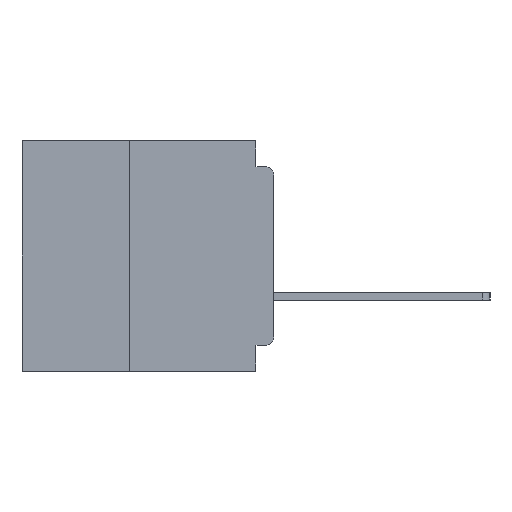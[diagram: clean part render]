
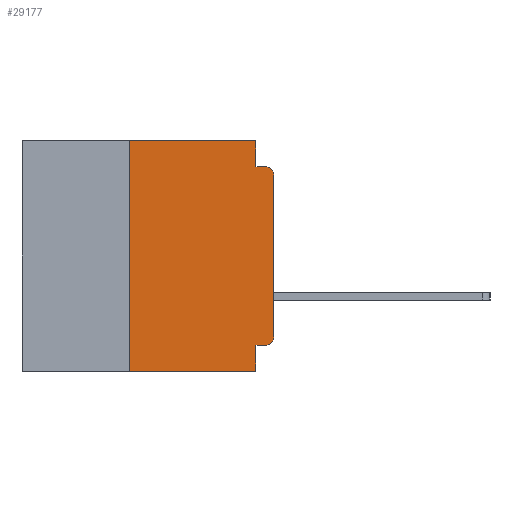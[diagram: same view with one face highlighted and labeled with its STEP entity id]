
A CAD part, left-side view. The second image highlights one B-rep face of the part: STEP entity #29177.
In plain terms, the highlighted planar face has unit normal (-1, 0, 0).
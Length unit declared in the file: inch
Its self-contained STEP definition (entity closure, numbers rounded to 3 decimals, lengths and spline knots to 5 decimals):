
#513 = LINE ( 'NONE', #43981, #28404 ) ;
#1409 = AXIS2_PLACEMENT_3D ( 'NONE', #6275, #32780, #10095 ) ;
#1496 = EDGE_CURVE ( 'NONE', #41549, #32029, #35087, .T. ) ;
#1542 = VERTEX_POINT ( 'NONE', #25859 ) ;
#1912 = VERTEX_POINT ( 'NONE', #33863 ) ;
#2236 = CARTESIAN_POINT ( 'NONE',  ( 0., 0.031, -0.355 ) ) ;
#2248 = ORIENTED_EDGE ( 'NONE', *, *, #45017, .T. ) ;
#3345 = VECTOR ( 'NONE', #23760, 39.37008 ) ;
#3802 = AXIS2_PLACEMENT_3D ( 'NONE', #3981, #30498, #7783 ) ;
#3981 = CARTESIAN_POINT ( 'NONE',  ( 0., 0.015, -0.34 ) ) ;
#4292 = CARTESIAN_POINT ( 'NONE',  ( 0., 0.437, 0. ) ) ;
#4428 = CARTESIAN_POINT ( 'NONE',  ( 0., 0., -0.34 ) ) ;
#5316 = CARTESIAN_POINT ( 'NONE',  ( 0., 0.015, -0.045 ) ) ;
#6275 = CARTESIAN_POINT ( 'NONE',  ( 0., 0.015, -0.06 ) ) ;
#6488 = CARTESIAN_POINT ( 'NONE',  ( 0., 0.25, -0.4 ) ) ;
#7777 = DIRECTION ( 'NONE',  ( 0., -1., 0. ) ) ;
#7783 = DIRECTION ( 'NONE',  ( 0., 0., -1. ) ) ;
#8103 = DIRECTION ( 'NONE',  ( 0., -1., 0. ) ) ;
#9694 = VERTEX_POINT ( 'NONE', #14199 ) ;
#10095 = DIRECTION ( 'NONE',  ( 0., 0., -1. ) ) ;
#10516 = LINE ( 'NONE', #4292, #39413 ) ;
#10620 = ORIENTED_EDGE ( 'NONE', *, *, #11874, .T. ) ;
#11874 = EDGE_CURVE ( 'NONE', #17379, #45347, #48627, .T. ) ;
#12501 = CARTESIAN_POINT ( 'NONE',  ( 0., 0.25, -0.4 ) ) ;
#12724 = DIRECTION ( 'NONE',  ( 0., -1., 0. ) ) ;
#12968 = ORIENTED_EDGE ( 'NONE', *, *, #31419, .T. ) ;
#14199 = CARTESIAN_POINT ( 'NONE',  ( 0., 0.031, -0.045 ) ) ;
#15267 = CARTESIAN_POINT ( 'NONE',  ( 0., 0., -0.045 ) ) ;
#15747 = PLANE ( 'NONE',  #40244 ) ;
#16006 = FACE_OUTER_BOUND ( 'NONE', #25511, .T. ) ;
#16915 = VERTEX_POINT ( 'NONE', #5316 ) ;
#17276 = ORIENTED_EDGE ( 'NONE', *, *, #38238, .F. ) ;
#17379 = VERTEX_POINT ( 'NONE', #4428 ) ;
#18901 = DIRECTION ( 'NONE',  ( 0., 1., 0. ) ) ;
#23354 = DIRECTION ( 'NONE',  ( 0., 0., -1. ) ) ;
#23691 = ORIENTED_EDGE ( 'NONE', *, *, #38173, .F. ) ;
#23760 = DIRECTION ( 'NONE',  ( 0., 0., 1. ) ) ;
#24192 = DIRECTION ( 'NONE',  ( 0., 0., -1. ) ) ;
#25119 = EDGE_CURVE ( 'NONE', #32029, #34562, #34734, .T. ) ;
#25344 = DIRECTION ( 'NONE',  ( 0., 0., -1. ) ) ;
#25511 = EDGE_LOOP ( 'NONE', ( #10620, #12968, #23691, #27265, #17276, #46495, #2248, #46539, #32540, #33720 ) ) ;
#25859 = CARTESIAN_POINT ( 'NONE',  ( 0., 0.031, 0. ) ) ;
#27265 = ORIENTED_EDGE ( 'NONE', *, *, #29520, .F. ) ;
#27590 = VECTOR ( 'NONE', #41375, 39.37008 ) ;
#28302 = CARTESIAN_POINT ( 'NONE',  ( 0., 0., -0.355 ) ) ;
#28404 = VECTOR ( 'NONE', #25344, 39.37008 ) ;
#29177 = ADVANCED_FACE ( 'NONE', ( #16006 ), #15747, .F. ) ;
#29520 = EDGE_CURVE ( 'NONE', #1542, #9694, #513, .T. ) ;
#29750 = CARTESIAN_POINT ( 'NONE',  ( 0., 0., -0.06 ) ) ;
#30498 = DIRECTION ( 'NONE',  ( -1., 0., 0. ) ) ;
#30633 = LINE ( 'NONE', #35356, #41716 ) ;
#31125 = CIRCLE ( 'NONE', #1409, 0.015 ) ;
#31168 = VECTOR ( 'NONE', #7777, 39.37008 ) ;
#31419 = EDGE_CURVE ( 'NONE', #45347, #16915, #31125, .T. ) ;
#32029 = VERTEX_POINT ( 'NONE', #2236 ) ;
#32540 = ORIENTED_EDGE ( 'NONE', *, *, #1496, .F. ) ;
#32780 = DIRECTION ( 'NONE',  ( -1., 0., 0. ) ) ;
#33720 = ORIENTED_EDGE ( 'NONE', *, *, #46046, .T. ) ;
#33863 = CARTESIAN_POINT ( 'NONE',  ( 0., 0.25, 0. ) ) ;
#34562 = VERTEX_POINT ( 'NONE', #36659 ) ;
#34734 = LINE ( 'NONE', #35379, #43492 ) ;
#35087 = LINE ( 'NONE', #28302, #41478 ) ;
#35356 = CARTESIAN_POINT ( 'NONE',  ( 0., 0.437, -0.4 ) ) ;
#35379 = CARTESIAN_POINT ( 'NONE',  ( 0., 0.031, -0.4 ) ) ;
#36659 = CARTESIAN_POINT ( 'NONE',  ( 0., 0.031, -0.4 ) ) ;
#37742 = EDGE_CURVE ( 'NONE', #42881, #1912, #43505, .T. ) ;
#38173 = EDGE_CURVE ( 'NONE', #9694, #16915, #41076, .T. ) ;
#38238 = EDGE_CURVE ( 'NONE', #1912, #1542, #10516, .T. ) ;
#39413 = VECTOR ( 'NONE', #8103, 39.37008 ) ;
#40244 = AXIS2_PLACEMENT_3D ( 'NONE', #42059, #45816, #23354 ) ;
#40973 = CARTESIAN_POINT ( 'NONE',  ( 0., 0.015, -0.355 ) ) ;
#40996 = CIRCLE ( 'NONE', #3802, 0.015 ) ;
#41076 = LINE ( 'NONE', #15267, #31168 ) ;
#41375 = DIRECTION ( 'NONE',  ( 0., 0., 1. ) ) ;
#41478 = VECTOR ( 'NONE', #18901, 39.37008 ) ;
#41549 = VERTEX_POINT ( 'NONE', #40973 ) ;
#41716 = VECTOR ( 'NONE', #12724, 39.37008 ) ;
#42059 = CARTESIAN_POINT ( 'NONE',  ( 0., 0.437, 0. ) ) ;
#42881 = VERTEX_POINT ( 'NONE', #6488 ) ;
#43492 = VECTOR ( 'NONE', #24192, 39.37008 ) ;
#43505 = LINE ( 'NONE', #12501, #3345 ) ;
#43981 = CARTESIAN_POINT ( 'NONE',  ( 0., 0.031, 0. ) ) ;
#45017 = EDGE_CURVE ( 'NONE', #42881, #34562, #30633, .T. ) ;
#45129 = CARTESIAN_POINT ( 'NONE',  ( 0., 0., 0. ) ) ;
#45347 = VERTEX_POINT ( 'NONE', #29750 ) ;
#45816 = DIRECTION ( 'NONE',  ( 1., 0., 0. ) ) ;
#46046 = EDGE_CURVE ( 'NONE', #41549, #17379, #40996, .T. ) ;
#46495 = ORIENTED_EDGE ( 'NONE', *, *, #37742, .F. ) ;
#46539 = ORIENTED_EDGE ( 'NONE', *, *, #25119, .F. ) ;
#48627 = LINE ( 'NONE', #45129, #27590 ) ;
